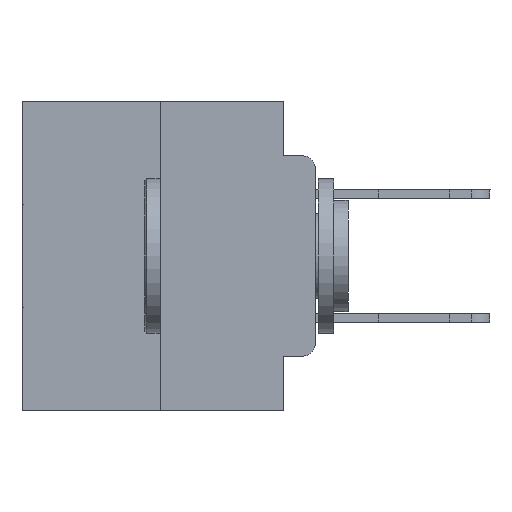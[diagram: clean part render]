
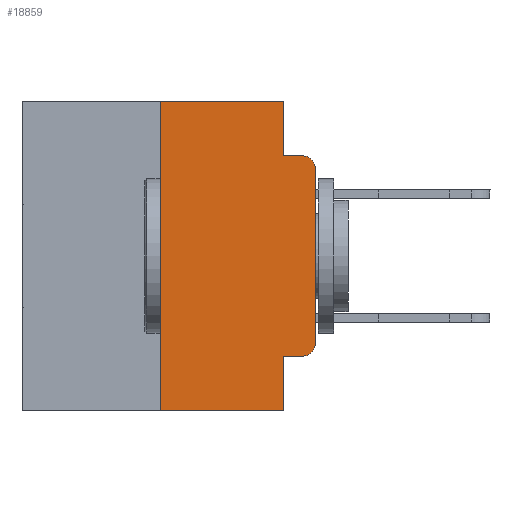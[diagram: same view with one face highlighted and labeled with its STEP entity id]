
A CAD part, left-side view. The second image highlights one B-rep face of the part: STEP entity #18859.
In plain terms, the highlighted planar face has unit normal (-1, 0, 0).
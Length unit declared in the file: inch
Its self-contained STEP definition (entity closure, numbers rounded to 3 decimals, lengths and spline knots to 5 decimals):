
#236 = CARTESIAN_POINT ( 'NONE',  ( 0., 0.051, -0.0885 ) ) ;
#295 = DIRECTION ( 'NONE',  ( 1., 0., 0. ) ) ;
#327 = VERTEX_POINT ( 'NONE', #26222 ) ;
#754 = VERTEX_POINT ( 'NONE', #2443 ) ;
#1123 = ORIENTED_EDGE ( 'NONE', *, *, #25738, .F. ) ;
#1394 = VERTEX_POINT ( 'NONE', #23373 ) ;
#1496 = VERTEX_POINT ( 'NONE', #9099 ) ;
#1851 = VERTEX_POINT ( 'NONE', #9373 ) ;
#1990 = DIRECTION ( 'NONE',  ( 0., 0., -1. ) ) ;
#2238 = VERTEX_POINT ( 'NONE', #10178 ) ;
#2443 = CARTESIAN_POINT ( 'NONE',  ( 0., 0.051, 0. ) ) ;
#2694 = CARTESIAN_POINT ( 'NONE',  ( 0., 0.051, 0. ) ) ;
#3487 = VECTOR ( 'NONE', #20368, 39.37008 ) ;
#3571 = LINE ( 'NONE', #12621, #11148 ) ;
#3830 = LINE ( 'NONE', #27862, #25611 ) ;
#4228 = ORIENTED_EDGE ( 'NONE', *, *, #24340, .F. ) ;
#4399 = CARTESIAN_POINT ( 'NONE',  ( 0., 0.02, -0.1085 ) ) ;
#4530 = VERTEX_POINT ( 'NONE', #16179 ) ;
#4725 = CARTESIAN_POINT ( 'NONE',  ( 0., 0., 0. ) ) ;
#5045 = ORIENTED_EDGE ( 'NONE', *, *, #21393, .T. ) ;
#5299 = VERTEX_POINT ( 'NONE', #15810 ) ;
#5842 = CARTESIAN_POINT ( 'NONE',  ( 0., 0.051, -0.4115 ) ) ;
#6466 = EDGE_CURVE ( 'NONE', #1851, #2238, #10529, .T. ) ;
#7427 = EDGE_CURVE ( 'NONE', #1496, #1394, #18901, .T. ) ;
#8116 = DIRECTION ( 'NONE',  ( 0., 0., -1. ) ) ;
#9099 = CARTESIAN_POINT ( 'NONE',  ( 0., 0., -0.1085 ) ) ;
#9158 = LINE ( 'NONE', #2694, #12511 ) ;
#9373 = CARTESIAN_POINT ( 'NONE',  ( 0., 0.02, -0.4115 ) ) ;
#10116 = CARTESIAN_POINT ( 'NONE',  ( 0., 0.02, -0.3915 ) ) ;
#10178 = CARTESIAN_POINT ( 'NONE',  ( 0., 0., -0.3915 ) ) ;
#10529 = CIRCLE ( 'NONE', #25231, 0.02 ) ;
#10555 = DIRECTION ( 'NONE',  ( -1., 0., 0. ) ) ;
#10596 = DIRECTION ( 'NONE',  ( 0., 0., 1. ) ) ;
#11040 = VECTOR ( 'NONE', #27309, 39.37008 ) ;
#11042 = DIRECTION ( 'NONE',  ( 0., 0., -1. ) ) ;
#11054 = VERTEX_POINT ( 'NONE', #23175 ) ;
#11148 = VECTOR ( 'NONE', #1990, 39.37008 ) ;
#11470 = DIRECTION ( 'NONE',  ( 0., -1., 0. ) ) ;
#12079 = EDGE_CURVE ( 'NONE', #19639, #1851, #18487, .T. ) ;
#12511 = VECTOR ( 'NONE', #11042, 39.37008 ) ;
#12595 = VECTOR ( 'NONE', #14319, 39.37008 ) ;
#12621 = CARTESIAN_POINT ( 'NONE',  ( 0., 0.051, 0. ) ) ;
#13396 = DIRECTION ( 'NONE',  ( 0., 0., -1. ) ) ;
#14319 = DIRECTION ( 'NONE',  ( 0., -1., 0. ) ) ;
#15020 = CARTESIAN_POINT ( 'NONE',  ( 0., 0.473, -0.5 ) ) ;
#15810 = CARTESIAN_POINT ( 'NONE',  ( 0., 0.051, -0.5 ) ) ;
#16179 = CARTESIAN_POINT ( 'NONE',  ( 0., 0.25, 0. ) ) ;
#16198 = LINE ( 'NONE', #4725, #11040 ) ;
#16562 = EDGE_CURVE ( 'NONE', #327, #4530, #3830, .T. ) ;
#17403 = FACE_OUTER_BOUND ( 'NONE', #25007, .T. ) ;
#17916 = LINE ( 'NONE', #236, #25938 ) ;
#18026 = VECTOR ( 'NONE', #19887, 39.37008 ) ;
#18216 = ORIENTED_EDGE ( 'NONE', *, *, #7427, .T. ) ;
#18466 = AXIS2_PLACEMENT_3D ( 'NONE', #4399, #26132, #24245 ) ;
#18487 = LINE ( 'NONE', #5842, #12595 ) ;
#18859 = ADVANCED_FACE ( 'NONE', ( #17403 ), #21884, .F. ) ;
#18901 = CIRCLE ( 'NONE', #18466, 0.02 ) ;
#19467 = EDGE_CURVE ( 'NONE', #2238, #1496, #16198, .T. ) ;
#19480 = ORIENTED_EDGE ( 'NONE', *, *, #6466, .T. ) ;
#19617 = ORIENTED_EDGE ( 'NONE', *, *, #22087, .F. ) ;
#19639 = VERTEX_POINT ( 'NONE', #23504 ) ;
#19887 = DIRECTION ( 'NONE',  ( 0., -1., 0. ) ) ;
#20134 = CARTESIAN_POINT ( 'NONE',  ( 0., 0.473, 0. ) ) ;
#20368 = DIRECTION ( 'NONE',  ( 0., -1., 0. ) ) ;
#21005 = ORIENTED_EDGE ( 'NONE', *, *, #16562, .F. ) ;
#21393 = EDGE_CURVE ( 'NONE', #327, #5299, #28416, .T. ) ;
#21630 = ORIENTED_EDGE ( 'NONE', *, *, #12079, .T. ) ;
#21884 = PLANE ( 'NONE',  #26629 ) ;
#22087 = EDGE_CURVE ( 'NONE', #19639, #5299, #3571, .T. ) ;
#22319 = EDGE_CURVE ( 'NONE', #754, #11054, #9158, .T. ) ;
#23175 = CARTESIAN_POINT ( 'NONE',  ( 0., 0.051, -0.0885 ) ) ;
#23373 = CARTESIAN_POINT ( 'NONE',  ( 0., 0.02, -0.0885 ) ) ;
#23504 = CARTESIAN_POINT ( 'NONE',  ( 0., 0.051, -0.4115 ) ) ;
#24150 = LINE ( 'NONE', #26470, #3487 ) ;
#24245 = DIRECTION ( 'NONE',  ( 0., 0., -1. ) ) ;
#24340 = EDGE_CURVE ( 'NONE', #11054, #1394, #17916, .T. ) ;
#24922 = ORIENTED_EDGE ( 'NONE', *, *, #22319, .F. ) ;
#25007 = EDGE_LOOP ( 'NONE', ( #26040, #18216, #4228, #24922, #1123, #21005, #5045, #19617, #21630, #19480 ) ) ;
#25231 = AXIS2_PLACEMENT_3D ( 'NONE', #10116, #10555, #8116 ) ;
#25611 = VECTOR ( 'NONE', #10596, 39.37008 ) ;
#25738 = EDGE_CURVE ( 'NONE', #4530, #754, #24150, .T. ) ;
#25938 = VECTOR ( 'NONE', #11470, 39.37008 ) ;
#26040 = ORIENTED_EDGE ( 'NONE', *, *, #19467, .T. ) ;
#26132 = DIRECTION ( 'NONE',  ( -1., 0., 0. ) ) ;
#26222 = CARTESIAN_POINT ( 'NONE',  ( 0., 0.25, -0.5 ) ) ;
#26470 = CARTESIAN_POINT ( 'NONE',  ( 0., 0.473, 0. ) ) ;
#26629 = AXIS2_PLACEMENT_3D ( 'NONE', #20134, #295, #13396 ) ;
#27309 = DIRECTION ( 'NONE',  ( 0., 0., 1. ) ) ;
#27862 = CARTESIAN_POINT ( 'NONE',  ( 0., 0.25, 0. ) ) ;
#28416 = LINE ( 'NONE', #15020, #18026 ) ;
